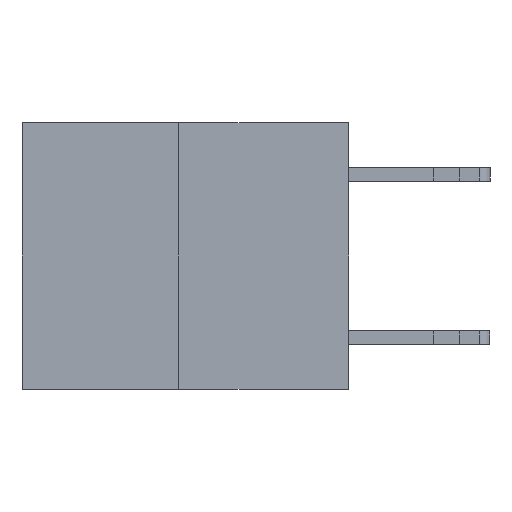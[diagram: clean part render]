
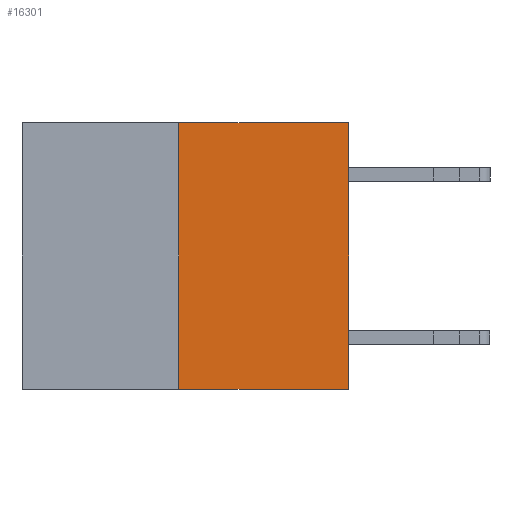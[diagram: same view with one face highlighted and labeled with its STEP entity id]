
A CAD part, left-side view. The second image highlights one B-rep face of the part: STEP entity #16301.
In plain terms, the highlighted planar face has unit normal (-1, 0, 0).
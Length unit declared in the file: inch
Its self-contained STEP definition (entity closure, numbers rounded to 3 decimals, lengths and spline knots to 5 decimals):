
#210 = LINE ( 'NONE', #7246, #15301 ) ;
#1165 = VECTOR ( 'NONE', #11039, 39.37008 ) ;
#1315 = VECTOR ( 'NONE', #14690, 39.37008 ) ;
#1380 = EDGE_CURVE ( 'NONE', #5198, #15052, #2967, .T. ) ;
#1591 = AXIS2_PLACEMENT_3D ( 'NONE', #17682, #10473, #13297 ) ;
#2165 = EDGE_LOOP ( 'NONE', ( #13783, #14657, #15952, #9652 ) ) ;
#2967 = LINE ( 'NONE', #3168, #18775 ) ;
#3168 = CARTESIAN_POINT ( 'NONE',  ( 0., 0., 0. ) ) ;
#3770 = CARTESIAN_POINT ( 'NONE',  ( 0., 0.6, 0. ) ) ;
#3805 = EDGE_CURVE ( 'NONE', #10228, #5198, #5186, .T. ) ;
#4191 = CARTESIAN_POINT ( 'NONE',  ( 0., 0.6, -0.49 ) ) ;
#4569 = DIRECTION ( 'NONE',  ( 0., 0., 1. ) ) ;
#5186 = LINE ( 'NONE', #4191, #1315 ) ;
#5195 = CARTESIAN_POINT ( 'NONE',  ( 0., 0.312, -0.49 ) ) ;
#5198 = VERTEX_POINT ( 'NONE', #13937 ) ;
#5657 = CARTESIAN_POINT ( 'NONE',  ( 0., 0., 0. ) ) ;
#6633 = LINE ( 'NONE', #3770, #1165 ) ;
#7246 = CARTESIAN_POINT ( 'NONE',  ( 0., 0.312, -0.49 ) ) ;
#8405 = FACE_OUTER_BOUND ( 'NONE', #2165, .T. ) ;
#9361 = EDGE_CURVE ( 'NONE', #10228, #17019, #210, .T. ) ;
#9652 = ORIENTED_EDGE ( 'NONE', *, *, #15388, .F. ) ;
#10228 = VERTEX_POINT ( 'NONE', #5195 ) ;
#10473 = DIRECTION ( 'NONE',  ( 1., 0., 0. ) ) ;
#11039 = DIRECTION ( 'NONE',  ( 0., -1., 0. ) ) ;
#11803 = PLANE ( 'NONE',  #1591 ) ;
#13297 = DIRECTION ( 'NONE',  ( 0., 0., -1. ) ) ;
#13783 = ORIENTED_EDGE ( 'NONE', *, *, #9361, .F. ) ;
#13937 = CARTESIAN_POINT ( 'NONE',  ( 0., 0., -0.49 ) ) ;
#14657 = ORIENTED_EDGE ( 'NONE', *, *, #3805, .T. ) ;
#14690 = DIRECTION ( 'NONE',  ( 0., -1., 0. ) ) ;
#14714 = DIRECTION ( 'NONE',  ( 0., 0., 1. ) ) ;
#15052 = VERTEX_POINT ( 'NONE', #5657 ) ;
#15301 = VECTOR ( 'NONE', #14714, 39.37008 ) ;
#15388 = EDGE_CURVE ( 'NONE', #17019, #15052, #6633, .T. ) ;
#15952 = ORIENTED_EDGE ( 'NONE', *, *, #1380, .T. ) ;
#16301 = ADVANCED_FACE ( 'NONE', ( #8405 ), #11803, .F. ) ;
#16350 = CARTESIAN_POINT ( 'NONE',  ( 0., 0.312, 0. ) ) ;
#17019 = VERTEX_POINT ( 'NONE', #16350 ) ;
#17682 = CARTESIAN_POINT ( 'NONE',  ( 0., 0.6, 0. ) ) ;
#18775 = VECTOR ( 'NONE', #4569, 39.37008 ) ;
